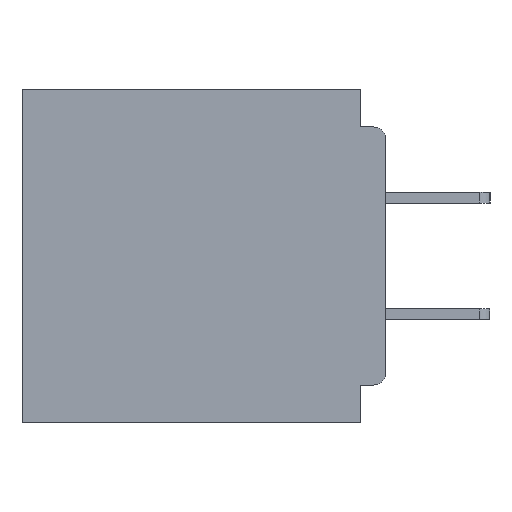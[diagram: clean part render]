
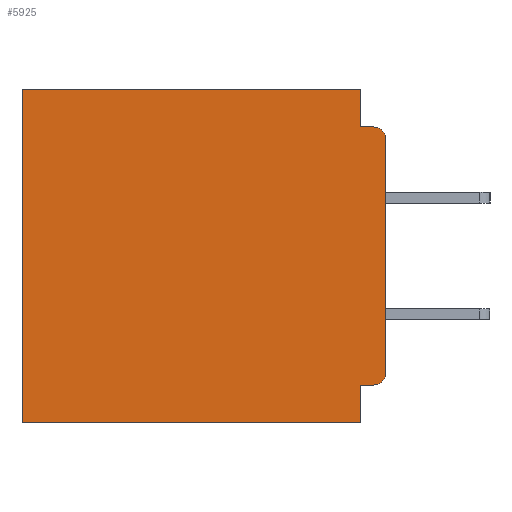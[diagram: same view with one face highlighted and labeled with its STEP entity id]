
A CAD part, left-side view. The second image highlights one B-rep face of the part: STEP entity #5925.
In plain terms, the highlighted planar face has unit normal (-1, 0, 0).
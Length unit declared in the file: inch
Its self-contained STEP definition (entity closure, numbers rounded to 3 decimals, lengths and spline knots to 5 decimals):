
#39 = VERTEX_POINT ( 'NONE', #32844 ) ;
#324 = VERTEX_POINT ( 'NONE', #23551 ) ;
#912 = CARTESIAN_POINT ( 'NONE',  ( 0.3, 0.437, 0. ) ) ;
#1596 = LINE ( 'NONE', #2673, #20924 ) ;
#2673 = CARTESIAN_POINT ( 'NONE',  ( 0.3, 0., -0.355 ) ) ;
#2821 = VECTOR ( 'NONE', #5645, 39.37008 ) ;
#3730 = DIRECTION ( 'NONE',  ( 0., 0., -1. ) ) ;
#4067 = ORIENTED_EDGE ( 'NONE', *, *, #12544, .T. ) ;
#4852 = VERTEX_POINT ( 'NONE', #45090 ) ;
#4912 = ORIENTED_EDGE ( 'NONE', *, *, #21596, .F. ) ;
#5385 = CARTESIAN_POINT ( 'NONE',  ( 0.3, 0.437, -0.4 ) ) ;
#5549 = EDGE_CURVE ( 'NONE', #22106, #28747, #21572, .T. ) ;
#5645 = DIRECTION ( 'NONE',  ( 0., 0., -1. ) ) ;
#5925 = ADVANCED_FACE ( 'NONE', ( #25102 ), #20282, .F. ) ;
#6507 = DIRECTION ( 'NONE',  ( 0., 1., 0. ) ) ;
#10770 = EDGE_CURVE ( 'NONE', #35069, #34838, #45242, .T. ) ;
#10820 = ORIENTED_EDGE ( 'NONE', *, *, #10770, .F. ) ;
#11396 = CARTESIAN_POINT ( 'NONE',  ( 0.3, 0., -0.34 ) ) ;
#12345 = EDGE_CURVE ( 'NONE', #34838, #324, #17772, .T. ) ;
#12544 = EDGE_CURVE ( 'NONE', #40227, #32202, #33842, .T. ) ;
#12670 = LINE ( 'NONE', #18643, #41888 ) ;
#13088 = LINE ( 'NONE', #47554, #2821 ) ;
#13687 = CIRCLE ( 'NONE', #15603, 0.015 ) ;
#15603 = AXIS2_PLACEMENT_3D ( 'NONE', #49440, #26794, #3730 ) ;
#16695 = CARTESIAN_POINT ( 'NONE',  ( 0.3, 0.031, 0. ) ) ;
#17441 = EDGE_CURVE ( 'NONE', #39, #324, #13687, .T. ) ;
#17772 = LINE ( 'NONE', #23024, #45646 ) ;
#18351 = CARTESIAN_POINT ( 'NONE',  ( 0.3, 0., 0. ) ) ;
#18643 = CARTESIAN_POINT ( 'NONE',  ( 0.3, 0., -0.4 ) ) ;
#19391 = CARTESIAN_POINT ( 'NONE',  ( 0.3, 0.015, -0.355 ) ) ;
#20186 = ORIENTED_EDGE ( 'NONE', *, *, #46860, .F. ) ;
#20282 = PLANE ( 'NONE',  #42171 ) ;
#20329 = CARTESIAN_POINT ( 'NONE',  ( 0.3, 0.015, -0.34 ) ) ;
#20924 = VECTOR ( 'NONE', #6507, 39.37008 ) ;
#21572 = LINE ( 'NONE', #38861, #40528 ) ;
#21596 = EDGE_CURVE ( 'NONE', #4852, #32768, #13088, .T. ) ;
#22106 = VERTEX_POINT ( 'NONE', #912 ) ;
#22195 = CARTESIAN_POINT ( 'NONE',  ( 0.3, 0.031, -0.4 ) ) ;
#22213 = DIRECTION ( 'NONE',  ( 0., 1., 0. ) ) ;
#22489 = DIRECTION ( 'NONE',  ( 0., 1., 0. ) ) ;
#23024 = CARTESIAN_POINT ( 'NONE',  ( 0.3, 0., -0.045 ) ) ;
#23551 = CARTESIAN_POINT ( 'NONE',  ( 0.3, 0.015, -0.045 ) ) ;
#23680 = ORIENTED_EDGE ( 'NONE', *, *, #40019, .F. ) ;
#24157 = DIRECTION ( 'NONE',  ( 0., 0., -1. ) ) ;
#24902 = EDGE_CURVE ( 'NONE', #39, #32202, #41804, .T. ) ;
#25102 = FACE_OUTER_BOUND ( 'NONE', #32237, .T. ) ;
#25785 = ORIENTED_EDGE ( 'NONE', *, *, #5549, .T. ) ;
#26648 = CARTESIAN_POINT ( 'NONE',  ( 0.3, 0.031, -0.045 ) ) ;
#26794 = DIRECTION ( 'NONE',  ( -1., 0., 0. ) ) ;
#27591 = LINE ( 'NONE', #18351, #36473 ) ;
#28747 = VERTEX_POINT ( 'NONE', #5385 ) ;
#30051 = DIRECTION ( 'NONE',  ( 0., 0., -1. ) ) ;
#31739 = VECTOR ( 'NONE', #40533, 39.37008 ) ;
#32202 = VERTEX_POINT ( 'NONE', #11396 ) ;
#32237 = EDGE_LOOP ( 'NONE', ( #33784, #43492, #47522, #10820, #36948, #25785, #20186, #4912, #23680, #4067 ) ) ;
#32768 = VERTEX_POINT ( 'NONE', #22195 ) ;
#32844 = CARTESIAN_POINT ( 'NONE',  ( 0.3, 0., -0.06 ) ) ;
#33354 = AXIS2_PLACEMENT_3D ( 'NONE', #20329, #46854, #24157 ) ;
#33784 = ORIENTED_EDGE ( 'NONE', *, *, #24902, .F. ) ;
#33842 = CIRCLE ( 'NONE', #33354, 0.015 ) ;
#34838 = VERTEX_POINT ( 'NONE', #26648 ) ;
#35069 = VERTEX_POINT ( 'NONE', #43200 ) ;
#35142 = VECTOR ( 'NONE', #43283, 39.37008 ) ;
#36473 = VECTOR ( 'NONE', #22213, 39.37008 ) ;
#36587 = DIRECTION ( 'NONE',  ( 1., 0., 0. ) ) ;
#36720 = CARTESIAN_POINT ( 'NONE',  ( 0.3, 0., -0.4 ) ) ;
#36948 = ORIENTED_EDGE ( 'NONE', *, *, #38763, .T. ) ;
#38763 = EDGE_CURVE ( 'NONE', #35069, #22106, #27591, .T. ) ;
#38861 = CARTESIAN_POINT ( 'NONE',  ( 0.3, 0.437, -0.4 ) ) ;
#40019 = EDGE_CURVE ( 'NONE', #40227, #4852, #1596, .T. ) ;
#40227 = VERTEX_POINT ( 'NONE', #19391 ) ;
#40528 = VECTOR ( 'NONE', #30051, 39.37008 ) ;
#40533 = DIRECTION ( 'NONE',  ( 0., 0., -1. ) ) ;
#41804 = LINE ( 'NONE', #36720, #31739 ) ;
#41888 = VECTOR ( 'NONE', #22489, 39.37008 ) ;
#42023 = DIRECTION ( 'NONE',  ( 0., 0., -1. ) ) ;
#42171 = AXIS2_PLACEMENT_3D ( 'NONE', #48699, #36587, #42023 ) ;
#43200 = CARTESIAN_POINT ( 'NONE',  ( 0.3, 0.031, 0. ) ) ;
#43283 = DIRECTION ( 'NONE',  ( 0., 0., -1. ) ) ;
#43492 = ORIENTED_EDGE ( 'NONE', *, *, #17441, .T. ) ;
#45090 = CARTESIAN_POINT ( 'NONE',  ( 0.3, 0.031, -0.355 ) ) ;
#45242 = LINE ( 'NONE', #16695, #35142 ) ;
#45646 = VECTOR ( 'NONE', #49488, 39.37008 ) ;
#46854 = DIRECTION ( 'NONE',  ( -1., 0., 0. ) ) ;
#46860 = EDGE_CURVE ( 'NONE', #32768, #28747, #12670, .T. ) ;
#47522 = ORIENTED_EDGE ( 'NONE', *, *, #12345, .F. ) ;
#47554 = CARTESIAN_POINT ( 'NONE',  ( 0.3, 0.031, -0.4 ) ) ;
#48699 = CARTESIAN_POINT ( 'NONE',  ( 0.3, 0., -0.4 ) ) ;
#49440 = CARTESIAN_POINT ( 'NONE',  ( 0.3, 0.015, -0.06 ) ) ;
#49488 = DIRECTION ( 'NONE',  ( 0., -1., 0. ) ) ;
